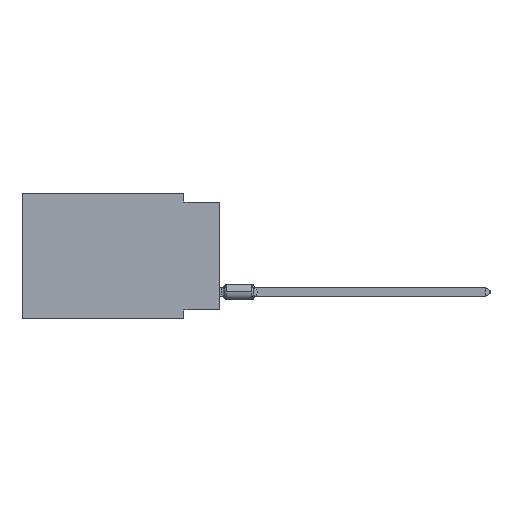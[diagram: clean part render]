
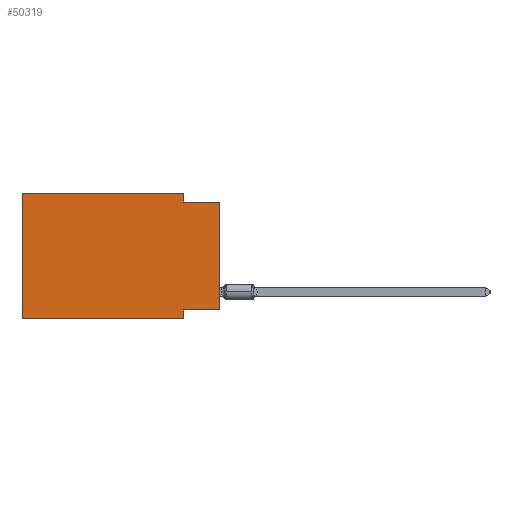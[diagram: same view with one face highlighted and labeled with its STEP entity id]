
A CAD part, left-side view. The second image highlights one B-rep face of the part: STEP entity #50319.
In plain terms, the highlighted planar face has unit normal (-1, 0, 0).
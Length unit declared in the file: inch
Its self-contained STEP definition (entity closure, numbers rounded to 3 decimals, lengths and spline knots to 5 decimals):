
#1450 = CARTESIAN_POINT ( 'NONE',  ( 0., 0., -0.325 ) ) ;
#2337 = DIRECTION ( 'NONE',  ( 0., 0., -1. ) ) ;
#3395 = DIRECTION ( 'NONE',  ( 0., -1., 0. ) ) ;
#3648 = ORIENTED_EDGE ( 'NONE', *, *, #7864, .T. ) ;
#5288 = CARTESIAN_POINT ( 'NONE',  ( 0., 0.55, 0. ) ) ;
#5797 = DIRECTION ( 'NONE',  ( 0., 0., -1. ) ) ;
#6427 = VERTEX_POINT ( 'NONE', #33665 ) ;
#6588 = CARTESIAN_POINT ( 'NONE',  ( 0., 0.55, -0.35 ) ) ;
#7864 = EDGE_CURVE ( 'NONE', #46404, #44852, #19381, .T. ) ;
#8406 = AXIS2_PLACEMENT_3D ( 'NONE', #21530, #25523, #50257 ) ;
#9574 = VERTEX_POINT ( 'NONE', #24634 ) ;
#10068 = VECTOR ( 'NONE', #3395, 39.37008 ) ;
#10413 = CARTESIAN_POINT ( 'NONE',  ( 0., 0.1, 0. ) ) ;
#10479 = VERTEX_POINT ( 'NONE', #14845 ) ;
#11272 = ORIENTED_EDGE ( 'NONE', *, *, #12118, .F. ) ;
#11567 = VERTEX_POINT ( 'NONE', #10413 ) ;
#12118 = EDGE_CURVE ( 'NONE', #35090, #13676, #48138, .T. ) ;
#12772 = DIRECTION ( 'NONE',  ( 0., -1., 0. ) ) ;
#13566 = ORIENTED_EDGE ( 'NONE', *, *, #25516, .F. ) ;
#13676 = VERTEX_POINT ( 'NONE', #28384 ) ;
#14845 = CARTESIAN_POINT ( 'NONE',  ( 0., 0.1, -0.325 ) ) ;
#14875 = VECTOR ( 'NONE', #12772, 39.37008 ) ;
#14971 = CARTESIAN_POINT ( 'NONE',  ( 0., 0.1, -0.35 ) ) ;
#15818 = VECTOR ( 'NONE', #31831, 39.37008 ) ;
#16173 = DIRECTION ( 'NONE',  ( 0., -1., 0. ) ) ;
#16651 = EDGE_CURVE ( 'NONE', #11567, #35090, #51336, .T. ) ;
#19381 = LINE ( 'NONE', #52634, #43436 ) ;
#19512 = CARTESIAN_POINT ( 'NONE',  ( 0., 0.1, -0.025 ) ) ;
#21176 = DIRECTION ( 'NONE',  ( 0., 0., 1. ) ) ;
#21530 = CARTESIAN_POINT ( 'NONE',  ( 0., 0.55, 0. ) ) ;
#21954 = LINE ( 'NONE', #46169, #26913 ) ;
#22051 = FACE_OUTER_BOUND ( 'NONE', #49422, .T. ) ;
#24634 = CARTESIAN_POINT ( 'NONE',  ( 0., 0.55, 0. ) ) ;
#24867 = EDGE_CURVE ( 'NONE', #9574, #11567, #45519, .T. ) ;
#25516 = EDGE_CURVE ( 'NONE', #46404, #9574, #48324, .T. ) ;
#25523 = DIRECTION ( 'NONE',  ( 1., 0., 0. ) ) ;
#25613 = ORIENTED_EDGE ( 'NONE', *, *, #24867, .F. ) ;
#26861 = CARTESIAN_POINT ( 'NONE',  ( 0., 0.1, 0. ) ) ;
#26913 = VECTOR ( 'NONE', #21176, 39.37008 ) ;
#28384 = CARTESIAN_POINT ( 'NONE',  ( 0., 0., -0.025 ) ) ;
#31089 = ORIENTED_EDGE ( 'NONE', *, *, #51954, .F. ) ;
#31328 = EDGE_CURVE ( 'NONE', #10479, #44852, #35366, .T. ) ;
#31831 = DIRECTION ( 'NONE',  ( 0., 0., 1. ) ) ;
#32628 = CARTESIAN_POINT ( 'NONE',  ( 0., 0.55, 0. ) ) ;
#33477 = ORIENTED_EDGE ( 'NONE', *, *, #16651, .F. ) ;
#33665 = CARTESIAN_POINT ( 'NONE',  ( 0., 0., -0.325 ) ) ;
#34288 = PLANE ( 'NONE',  #8406 ) ;
#34909 = VECTOR ( 'NONE', #2337, 39.37008 ) ;
#35090 = VERTEX_POINT ( 'NONE', #19512 ) ;
#35366 = LINE ( 'NONE', #42818, #50135 ) ;
#39209 = VECTOR ( 'NONE', #41440, 39.37008 ) ;
#40046 = EDGE_CURVE ( 'NONE', #6427, #13676, #21954, .T. ) ;
#40168 = CARTESIAN_POINT ( 'NONE',  ( 0., 0., -0.025 ) ) ;
#41440 = DIRECTION ( 'NONE',  ( 0., 1., 0. ) ) ;
#42818 = CARTESIAN_POINT ( 'NONE',  ( 0., 0.1, -0.35 ) ) ;
#43436 = VECTOR ( 'NONE', #16173, 39.37008 ) ;
#44852 = VERTEX_POINT ( 'NONE', #14971 ) ;
#45251 = ORIENTED_EDGE ( 'NONE', *, *, #31328, .F. ) ;
#45378 = ORIENTED_EDGE ( 'NONE', *, *, #40046, .T. ) ;
#45423 = LINE ( 'NONE', #1450, #39209 ) ;
#45519 = LINE ( 'NONE', #5288, #14875 ) ;
#46169 = CARTESIAN_POINT ( 'NONE',  ( 0., 0., 0. ) ) ;
#46404 = VERTEX_POINT ( 'NONE', #6588 ) ;
#48138 = LINE ( 'NONE', #40168, #10068 ) ;
#48324 = LINE ( 'NONE', #32628, #15818 ) ;
#49422 = EDGE_LOOP ( 'NONE', ( #45378, #11272, #33477, #25613, #13566, #3648, #45251, #31089 ) ) ;
#50135 = VECTOR ( 'NONE', #5797, 39.37008 ) ;
#50257 = DIRECTION ( 'NONE',  ( 0., 0., -1. ) ) ;
#50319 = ADVANCED_FACE ( 'NONE', ( #22051 ), #34288, .F. ) ;
#51336 = LINE ( 'NONE', #26861, #34909 ) ;
#51954 = EDGE_CURVE ( 'NONE', #6427, #10479, #45423, .T. ) ;
#52634 = CARTESIAN_POINT ( 'NONE',  ( 0., 0.55, -0.35 ) ) ;
